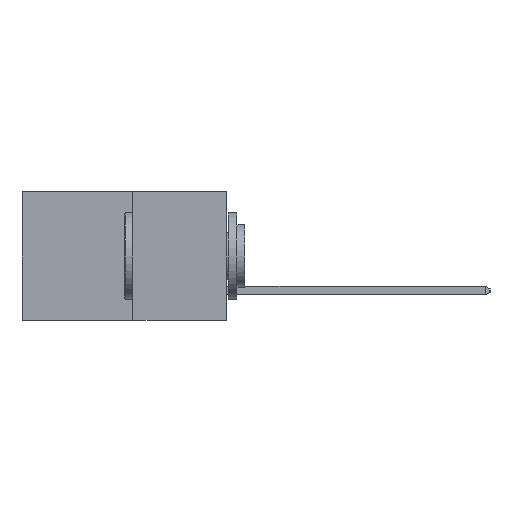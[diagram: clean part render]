
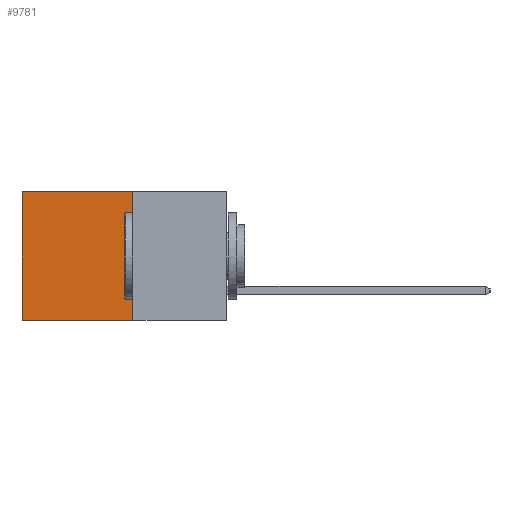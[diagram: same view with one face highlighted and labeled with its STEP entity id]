
A CAD part, left-side view. The second image highlights one B-rep face of the part: STEP entity #9781.
In plain terms, the highlighted planar face has unit normal (-1, 0, 0).
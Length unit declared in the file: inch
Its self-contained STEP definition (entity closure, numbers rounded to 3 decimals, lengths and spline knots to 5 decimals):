
#482 = VERTEX_POINT ( 'NONE', #26681 ) ;
#699 = CARTESIAN_POINT ( 'NONE',  ( 0.277, 0.27, 0. ) ) ;
#1470 = EDGE_LOOP ( 'NONE', ( #20410, #28161, #26734, #12661 ) ) ;
#2971 = DIRECTION ( 'NONE',  ( 0., 1., 0. ) ) ;
#5032 = FACE_OUTER_BOUND ( 'NONE', #1470, .T. ) ;
#6278 = CARTESIAN_POINT ( 'NONE',  ( 0.277, 0.27, -0.37 ) ) ;
#6462 = PLANE ( 'NONE',  #11481 ) ;
#6620 = VECTOR ( 'NONE', #20259, 39.37008 ) ;
#6629 = CARTESIAN_POINT ( 'NONE',  ( 0.277, 0.59, -0.37 ) ) ;
#7072 = VERTEX_POINT ( 'NONE', #25815 ) ;
#8118 = EDGE_CURVE ( 'NONE', #8657, #7072, #28162, .T. ) ;
#8657 = VERTEX_POINT ( 'NONE', #11502 ) ;
#8698 = DIRECTION ( 'NONE',  ( 1., 0., 0. ) ) ;
#8869 = DIRECTION ( 'NONE',  ( 0., 0., -1. ) ) ;
#9781 = ADVANCED_FACE ( 'NONE', ( #5032 ), #6462, .F. ) ;
#10472 = VECTOR ( 'NONE', #2971, 39.37008 ) ;
#11121 = LINE ( 'NONE', #6278, #26013 ) ;
#11481 = AXIS2_PLACEMENT_3D ( 'NONE', #22018, #8698, #24245 ) ;
#11502 = CARTESIAN_POINT ( 'NONE',  ( 0.277, 0.27, 0. ) ) ;
#12233 = VERTEX_POINT ( 'NONE', #23761 ) ;
#12661 = ORIENTED_EDGE ( 'NONE', *, *, #8118, .T. ) ;
#18003 = CARTESIAN_POINT ( 'NONE',  ( 0.277, 0.27, -0.37 ) ) ;
#19516 = VECTOR ( 'NONE', #8869, 39.37008 ) ;
#19931 = EDGE_CURVE ( 'NONE', #7072, #12233, #20214, .T. ) ;
#20214 = LINE ( 'NONE', #6629, #19516 ) ;
#20259 = DIRECTION ( 'NONE',  ( 0., 1., 0. ) ) ;
#20410 = ORIENTED_EDGE ( 'NONE', *, *, #19931, .T. ) ;
#21144 = EDGE_CURVE ( 'NONE', #8657, #482, #11121, .T. ) ;
#22018 = CARTESIAN_POINT ( 'NONE',  ( 0.277, 0.27, -0.37 ) ) ;
#23761 = CARTESIAN_POINT ( 'NONE',  ( 0.277, 0.59, -0.37 ) ) ;
#24245 = DIRECTION ( 'NONE',  ( 0., 0., -1. ) ) ;
#25041 = LINE ( 'NONE', #18003, #6620 ) ;
#25815 = CARTESIAN_POINT ( 'NONE',  ( 0.277, 0.59, 0. ) ) ;
#26013 = VECTOR ( 'NONE', #28512, 39.37008 ) ;
#26681 = CARTESIAN_POINT ( 'NONE',  ( 0.277, 0.27, -0.37 ) ) ;
#26734 = ORIENTED_EDGE ( 'NONE', *, *, #21144, .F. ) ;
#26776 = EDGE_CURVE ( 'NONE', #482, #12233, #25041, .T. ) ;
#28161 = ORIENTED_EDGE ( 'NONE', *, *, #26776, .F. ) ;
#28162 = LINE ( 'NONE', #699, #10472 ) ;
#28512 = DIRECTION ( 'NONE',  ( 0., 0., -1. ) ) ;
